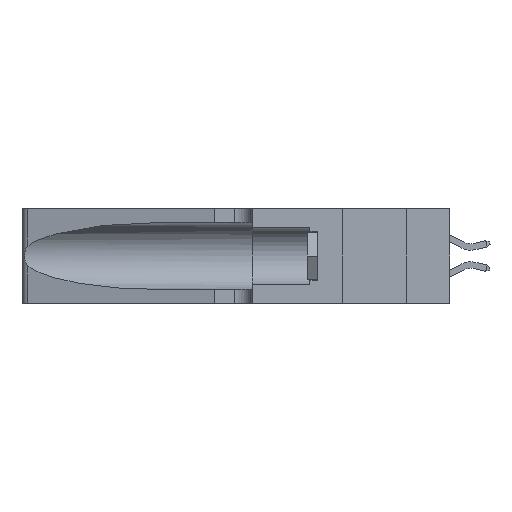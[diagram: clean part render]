
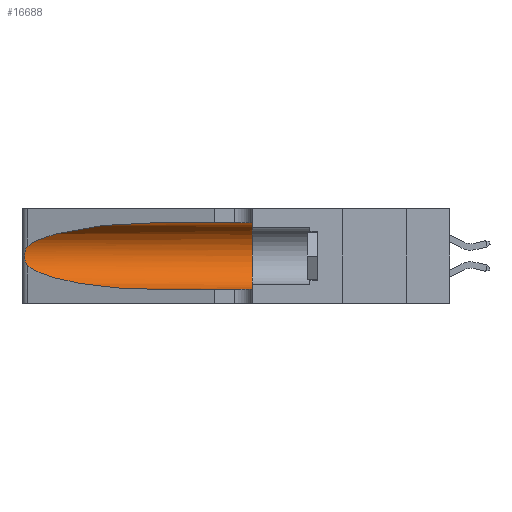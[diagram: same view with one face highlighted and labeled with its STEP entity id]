
A CAD part, left-side view. The second image highlights one B-rep face of the part: STEP entity #16688.
In plain terms, the highlighted cylindrical face has radius 3.308 mm (diameter 6.617 mm), a partial arc.
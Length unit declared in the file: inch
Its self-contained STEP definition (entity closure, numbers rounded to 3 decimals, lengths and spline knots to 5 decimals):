
#1705 =( BOUNDED_CURVE ( )  B_SPLINE_CURVE ( 3, ( #9515, #12381, #7131, #29547 ),
 .UNSPECIFIED., .F., .F. ) 
 B_SPLINE_CURVE_WITH_KNOTS ( ( 4, 4 ),
 ( 1.5708, 2.84003 ),
 .UNSPECIFIED. ) 
 CURVE ( )  GEOMETRIC_REPRESENTATION_ITEM ( )  RATIONAL_B_SPLINE_CURVE ( ( 1., 0.87, 0.87, 1. ) ) 
 REPRESENTATION_ITEM ( '' )  );
#1765 = AXIS2_PLACEMENT_3D ( 'NONE', #24832, #18780, #13505 ) ;
#1875 = CARTESIAN_POINT ( 'NONE',  ( 0.26075, 1.23896, 0.178 ) ) ;
#2352 = EDGE_CURVE ( 'NONE', #26419, #27648, #14787, .T. ) ;
#3537 = VERTEX_POINT ( 'NONE', #25817 ) ;
#4453 = DIRECTION ( 'NONE',  ( 0., -1., 0. ) ) ;
#4705 = CARTESIAN_POINT ( 'NONE',  ( 0.25856, 1.23593, 0.16098 ) ) ;
#5238 = VERTEX_POINT ( 'NONE', #36325 ) ;
#6379 = CARTESIAN_POINT ( 'NONE',  ( 0.1305, 0.35, 0.05475 ) ) ;
#7131 = CARTESIAN_POINT ( 'NONE',  ( 0.2373, 1.15595, 0.28018 ) ) ;
#7322 = CARTESIAN_POINT ( 'NONE',  ( 0.25639, 1.23184, 0.21858 ) ) ;
#7528 = CARTESIAN_POINT ( 'NONE',  ( 0.1305, 0.72297, 0.31525 ) ) ;
#7742 = ORIENTED_EDGE ( 'NONE', *, *, #32445, .T. ) ;
#7906 = CYLINDRICAL_SURFACE ( 'NONE', #35704, 0.13025 ) ;
#8911 = DIRECTION ( 'NONE',  ( 0., -1., 0. ) ) ;
#9330 = CARTESIAN_POINT ( 'NONE',  ( 0.2373, 1.15595, 0.08982 ) ) ;
#9515 = CARTESIAN_POINT ( 'NONE',  ( 0.1305, 0.72297, 0.31525 ) ) ;
#9786 = EDGE_CURVE ( 'NONE', #26419, #29315, #1705, .T. ) ;
#10238 = DIRECTION ( 'NONE',  ( 0., 0., -1. ) ) ;
#10287 = CARTESIAN_POINT ( 'NONE',  ( 0.26018, 1.23835, 0.19895 ) ) ;
#10663 = ORIENTED_EDGE ( 'NONE', *, *, #2352, .F. ) ;
#11745 = VERTEX_POINT ( 'NONE', #6379 ) ;
#12381 = CARTESIAN_POINT ( 'NONE',  ( 0.18966, 0.96281, 0.31525 ) ) ;
#12881 = DIRECTION ( 'NONE',  ( 0., -1., 0. ) ) ;
#13505 = DIRECTION ( 'NONE',  ( 0., 0., 1. ) ) ;
#13741 =( BOUNDED_CURVE ( )  B_SPLINE_CURVE ( 3, ( #23250, #9330, #26143, #14660 ),
 .UNSPECIFIED., .F., .T. ) 
 B_SPLINE_CURVE_WITH_KNOTS ( ( 4, 4 ),
 ( 3.44316, 4.71239 ),
 .UNSPECIFIED. ) 
 CURVE ( )  GEOMETRIC_REPRESENTATION_ITEM ( )  RATIONAL_B_SPLINE_CURVE ( ( 1., 0.87, 0.87, 1. ) ) 
 REPRESENTATION_ITEM ( '' )  );
#13868 = VECTOR ( 'NONE', #8911, 39.37008 ) ;
#13880 = CARTESIAN_POINT ( 'NONE',  ( 0.25487, 1.22718, 0.14631 ) ) ;
#14315 = ORIENTED_EDGE ( 'NONE', *, *, #20650, .T. ) ;
#14660 = CARTESIAN_POINT ( 'NONE',  ( 0.1305, 0.72297, 0.05475 ) ) ;
#14787 = LINE ( 'NONE', #17249, #13868 ) ;
#15258 = LINE ( 'NONE', #35525, #18393 ) ;
#16688 = ADVANCED_FACE ( 'NONE', ( #30597 ), #7906, .F. ) ;
#17249 = CARTESIAN_POINT ( 'NONE',  ( 0.1305, 1.61858, 0.31525 ) ) ;
#18393 = VECTOR ( 'NONE', #4453, 39.37008 ) ;
#18780 = DIRECTION ( 'NONE',  ( 0., 1., 0. ) ) ;
#18787 = CARTESIAN_POINT ( 'NONE',  ( 0.25787, 1.23484, 0.2124 ) ) ;
#18802 = B_SPLINE_CURVE_WITH_KNOTS ( 'NONE', 3,
 ( #35656, #24361, #7322, #18787, #27370, #10287, #30207, #1875, #21750, #4705, #24596, #30922, #31158, #13880 ),
 .UNSPECIFIED., .F., .F.,
 ( 4, 2, 2, 2, 2, 2, 4 ),
 ( 0., 0.00027, 0.00053, 0.00107, 0.0016, 0.00187, 0.00214 ),
 .UNSPECIFIED. ) ;
#20650 = EDGE_CURVE ( 'NONE', #3537, #11745, #15258, .T. ) ;
#21750 = CARTESIAN_POINT ( 'NONE',  ( 0.26017, 1.23833, 0.17102 ) ) ;
#23250 = CARTESIAN_POINT ( 'NONE',  ( 0.25487, 1.22718, 0.14631 ) ) ;
#24361 = CARTESIAN_POINT ( 'NONE',  ( 0.25555, 1.22994, 0.2215 ) ) ;
#24596 = CARTESIAN_POINT ( 'NONE',  ( 0.25789, 1.23486, 0.15765 ) ) ;
#24804 = CARTESIAN_POINT ( 'NONE',  ( 0.25487, 1.22718, 0.22369 ) ) ;
#24832 = CARTESIAN_POINT ( 'NONE',  ( 0.1305, 0.35, 0.185 ) ) ;
#25817 = CARTESIAN_POINT ( 'NONE',  ( 0.1305, 0.72297, 0.05475 ) ) ;
#26143 = CARTESIAN_POINT ( 'NONE',  ( 0.18966, 0.96281, 0.05475 ) ) ;
#26419 = VERTEX_POINT ( 'NONE', #7528 ) ;
#26527 = ORIENTED_EDGE ( 'NONE', *, *, #30710, .F. ) ;
#27370 = CARTESIAN_POINT ( 'NONE',  ( 0.25854, 1.2359, 0.20912 ) ) ;
#27648 = VERTEX_POINT ( 'NONE', #29496 ) ;
#27816 = ORIENTED_EDGE ( 'NONE', *, *, #27838, .T. ) ;
#27838 = EDGE_CURVE ( 'NONE', #29315, #5238, #18802, .T. ) ;
#28733 = ORIENTED_EDGE ( 'NONE', *, *, #9786, .T. ) ;
#29315 = VERTEX_POINT ( 'NONE', #24804 ) ;
#29496 = CARTESIAN_POINT ( 'NONE',  ( 0.1305, 0.35, 0.31525 ) ) ;
#29547 = CARTESIAN_POINT ( 'NONE',  ( 0.25487, 1.22718, 0.22369 ) ) ;
#29612 = EDGE_LOOP ( 'NONE', ( #28733, #27816, #7742, #14315, #26527, #10663 ) ) ;
#30207 = CARTESIAN_POINT ( 'NONE',  ( 0.26075, 1.23896, 0.19203 ) ) ;
#30597 = FACE_OUTER_BOUND ( 'NONE', #29612, .T. ) ;
#30710 = EDGE_CURVE ( 'NONE', #27648, #11745, #33009, .T. ) ;
#30922 = CARTESIAN_POINT ( 'NONE',  ( 0.25639, 1.23186, 0.15144 ) ) ;
#31158 = CARTESIAN_POINT ( 'NONE',  ( 0.25555, 1.22993, 0.14849 ) ) ;
#32445 = EDGE_CURVE ( 'NONE', #5238, #3537, #13741, .T. ) ;
#32632 = CARTESIAN_POINT ( 'NONE',  ( 0.1305, 1.61858, 0.185 ) ) ;
#33009 = CIRCLE ( 'NONE', #1765, 0.13025 ) ;
#35525 = CARTESIAN_POINT ( 'NONE',  ( 0.1305, 1.61858, 0.05475 ) ) ;
#35656 = CARTESIAN_POINT ( 'NONE',  ( 0.25487, 1.22718, 0.22369 ) ) ;
#35704 = AXIS2_PLACEMENT_3D ( 'NONE', #32632, #12881, #10238 ) ;
#36325 = CARTESIAN_POINT ( 'NONE',  ( 0.25487, 1.22718, 0.14631 ) ) ;
